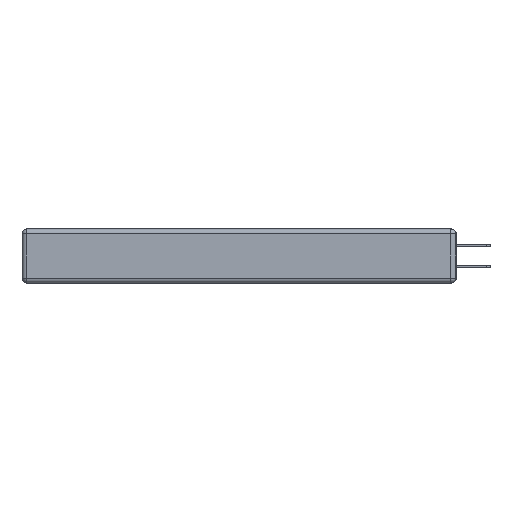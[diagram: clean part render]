
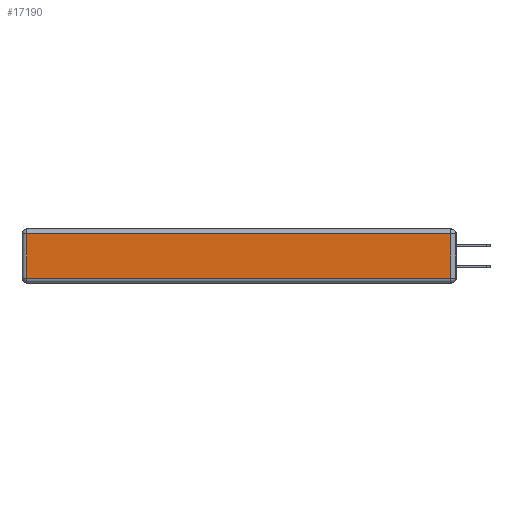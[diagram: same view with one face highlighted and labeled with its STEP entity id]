
A CAD part, left-side view. The second image highlights one B-rep face of the part: STEP entity #17190.
In plain terms, the highlighted planar face has unit normal (-1, 0, 0).
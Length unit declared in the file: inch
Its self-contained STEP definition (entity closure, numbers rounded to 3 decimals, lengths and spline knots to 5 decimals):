
#284 = CARTESIAN_POINT ( 'NONE',  ( 0., 0.03, -0.313 ) ) ;
#802 = EDGE_CURVE ( 'NONE', #14199, #10814, #2692, .T. ) ;
#1422 = VECTOR ( 'NONE', #19940, 39.37008 ) ;
#1467 = VERTEX_POINT ( 'NONE', #7639 ) ;
#2692 = LINE ( 'NONE', #13400, #1422 ) ;
#2887 = LINE ( 'NONE', #15843, #13129 ) ;
#3524 = CARTESIAN_POINT ( 'NONE',  ( 0., 2.72, -0.343 ) ) ;
#4420 = LINE ( 'NONE', #9479, #10798 ) ;
#5064 = DIRECTION ( 'NONE',  ( 0., 0., -1. ) ) ;
#5478 = LINE ( 'NONE', #3524, #11608 ) ;
#5781 = EDGE_LOOP ( 'NONE', ( #10876, #12949, #19778, #18305 ) ) ;
#7168 = EDGE_CURVE ( 'NONE', #7342, #1467, #5478, .T. ) ;
#7342 = VERTEX_POINT ( 'NONE', #16750 ) ;
#7639 = CARTESIAN_POINT ( 'NONE',  ( 0., 2.72, -0.313 ) ) ;
#8069 = PLANE ( 'NONE',  #20959 ) ;
#8128 = DIRECTION ( 'NONE',  ( 0., 0., 1. ) ) ;
#9420 = DIRECTION ( 'NONE',  ( 0., 1., 0. ) ) ;
#9479 = CARTESIAN_POINT ( 'NONE',  ( 0., 2.75, -0.03 ) ) ;
#10798 = VECTOR ( 'NONE', #9420, 39.37008 ) ;
#10814 = VERTEX_POINT ( 'NONE', #17858 ) ;
#10876 = ORIENTED_EDGE ( 'NONE', *, *, #13346, .T. ) ;
#11608 = VECTOR ( 'NONE', #5064, 39.37008 ) ;
#11649 = DIRECTION ( 'NONE',  ( -1., 0., 0. ) ) ;
#12584 = DIRECTION ( 'NONE',  ( 0., -1., 0. ) ) ;
#12949 = ORIENTED_EDGE ( 'NONE', *, *, #802, .T. ) ;
#13129 = VECTOR ( 'NONE', #12584, 39.37008 ) ;
#13346 = EDGE_CURVE ( 'NONE', #1467, #14199, #2887, .T. ) ;
#13400 = CARTESIAN_POINT ( 'NONE',  ( 0., 0.03, -0.343 ) ) ;
#14199 = VERTEX_POINT ( 'NONE', #284 ) ;
#15843 = CARTESIAN_POINT ( 'NONE',  ( 0., 0., -0.313 ) ) ;
#16529 = CARTESIAN_POINT ( 'NONE',  ( 0., 0., -0.343 ) ) ;
#16750 = CARTESIAN_POINT ( 'NONE',  ( 0., 2.72, -0.03 ) ) ;
#16780 = FACE_OUTER_BOUND ( 'NONE', #5781, .T. ) ;
#17069 = EDGE_CURVE ( 'NONE', #10814, #7342, #4420, .T. ) ;
#17190 = ADVANCED_FACE ( 'NONE', ( #16780 ), #8069, .T. ) ;
#17858 = CARTESIAN_POINT ( 'NONE',  ( 0., 0.03, -0.03 ) ) ;
#18305 = ORIENTED_EDGE ( 'NONE', *, *, #7168, .T. ) ;
#19778 = ORIENTED_EDGE ( 'NONE', *, *, #17069, .T. ) ;
#19940 = DIRECTION ( 'NONE',  ( 0., 0., 1. ) ) ;
#20959 = AXIS2_PLACEMENT_3D ( 'NONE', #16529, #11649, #8128 ) ;
